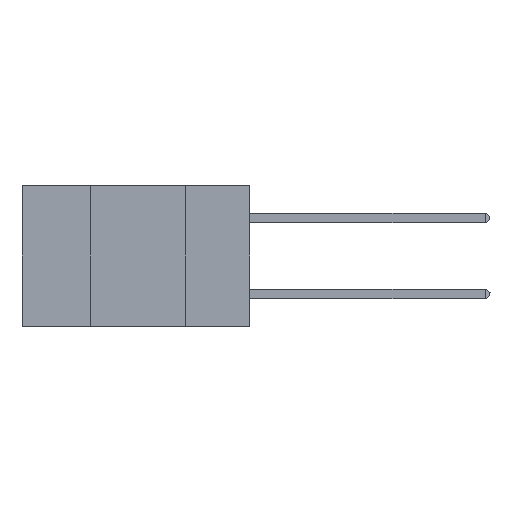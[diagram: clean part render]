
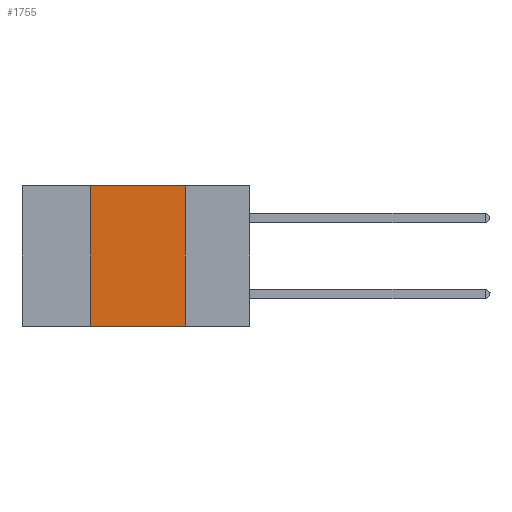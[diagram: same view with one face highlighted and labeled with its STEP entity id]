
A CAD part, left-side view. The second image highlights one B-rep face of the part: STEP entity #1755.
In plain terms, the highlighted planar face has unit normal (-1, 0, 0).
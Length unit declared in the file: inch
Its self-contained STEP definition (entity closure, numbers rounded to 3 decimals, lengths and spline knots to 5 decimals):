
#599 = DIRECTION ( 'NONE',  ( 1., 0., 0. ) ) ;
#1531 = CARTESIAN_POINT ( 'NONE',  ( 0., 0.17, 0. ) ) ;
#1755 = ADVANCED_FACE ( 'NONE', ( #11943 ), #23129, .F. ) ;
#1990 = CARTESIAN_POINT ( 'NONE',  ( 0., 0.17, -0.37 ) ) ;
#2403 = VECTOR ( 'NONE', #18615, 39.37008 ) ;
#6157 = LINE ( 'NONE', #31856, #14518 ) ;
#6596 = EDGE_CURVE ( 'NONE', #22113, #25062, #11353, .T. ) ;
#6620 = AXIS2_PLACEMENT_3D ( 'NONE', #20672, #599, #23316 ) ;
#8759 = DIRECTION ( 'NONE',  ( 0., -1., 0. ) ) ;
#9160 = CARTESIAN_POINT ( 'NONE',  ( 0., 0.42, 0. ) ) ;
#10051 = LINE ( 'NONE', #32793, #2403 ) ;
#10145 = ORIENTED_EDGE ( 'NONE', *, *, #6596, .T. ) ;
#10688 = EDGE_CURVE ( 'NONE', #22113, #33306, #18262, .T. ) ;
#11351 = ORIENTED_EDGE ( 'NONE', *, *, #10688, .F. ) ;
#11353 = LINE ( 'NONE', #36682, #28330 ) ;
#11943 = FACE_OUTER_BOUND ( 'NONE', #27993, .T. ) ;
#14518 = VECTOR ( 'NONE', #8759, 39.37008 ) ;
#18262 = LINE ( 'NONE', #9160, #23783 ) ;
#18615 = DIRECTION ( 'NONE',  ( 0., 0., -1. ) ) ;
#20672 = CARTESIAN_POINT ( 'NONE',  ( 0., 0.6, 0. ) ) ;
#22113 = VERTEX_POINT ( 'NONE', #25618 ) ;
#22520 = DIRECTION ( 'NONE',  ( 0., -1., 0. ) ) ;
#23129 = PLANE ( 'NONE',  #6620 ) ;
#23316 = DIRECTION ( 'NONE',  ( 0., 0., -1. ) ) ;
#23783 = VECTOR ( 'NONE', #32261, 39.37008 ) ;
#24312 = ORIENTED_EDGE ( 'NONE', *, *, #30757, .F. ) ;
#25062 = VERTEX_POINT ( 'NONE', #1990 ) ;
#25618 = CARTESIAN_POINT ( 'NONE',  ( 0., 0.42, -0.37 ) ) ;
#26047 = EDGE_CURVE ( 'NONE', #30453, #25062, #10051, .T. ) ;
#26922 = CARTESIAN_POINT ( 'NONE',  ( 0., 0.42, 0. ) ) ;
#27993 = EDGE_LOOP ( 'NONE', ( #35172, #24312, #11351, #10145 ) ) ;
#28330 = VECTOR ( 'NONE', #22520, 39.37008 ) ;
#30453 = VERTEX_POINT ( 'NONE', #1531 ) ;
#30757 = EDGE_CURVE ( 'NONE', #33306, #30453, #6157, .T. ) ;
#31856 = CARTESIAN_POINT ( 'NONE',  ( 0., 0.6, 0. ) ) ;
#32261 = DIRECTION ( 'NONE',  ( 0., 0., 1. ) ) ;
#32793 = CARTESIAN_POINT ( 'NONE',  ( 0., 0.17, 0. ) ) ;
#33306 = VERTEX_POINT ( 'NONE', #26922 ) ;
#35172 = ORIENTED_EDGE ( 'NONE', *, *, #26047, .F. ) ;
#36682 = CARTESIAN_POINT ( 'NONE',  ( 0., 0.6, -0.37 ) ) ;
